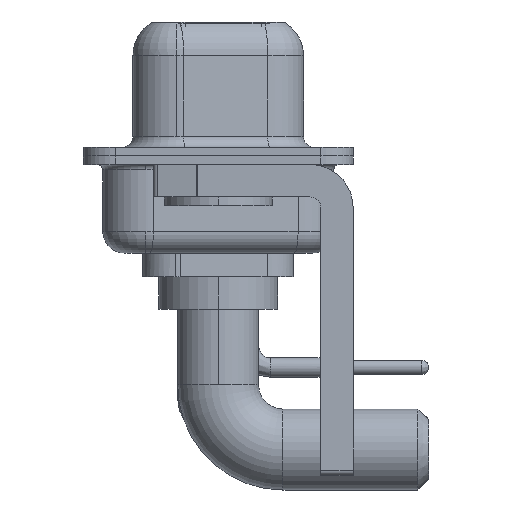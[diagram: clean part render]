
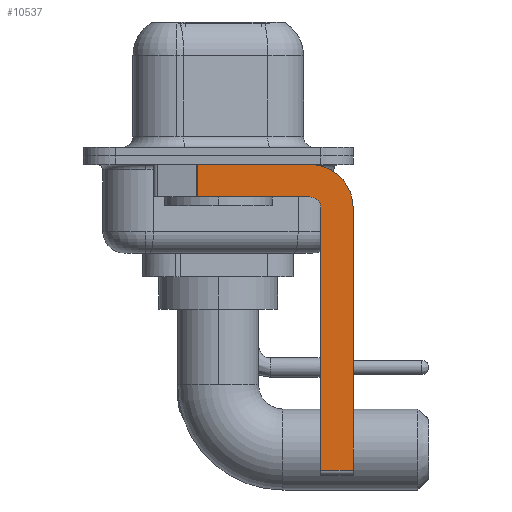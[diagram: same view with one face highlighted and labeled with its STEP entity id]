
A CAD part, left-side view. The second image highlights one B-rep face of the part: STEP entity #10537.
In plain terms, the highlighted planar face has unit normal (-1, 0, 0).
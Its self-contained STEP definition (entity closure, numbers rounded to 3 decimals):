
#95 = DIRECTION ( 'NONE',  ( 0., 0., -1. ) ) ;
#140 = VERTEX_POINT ( 'NONE', #16661 ) ;
#276 = CARTESIAN_POINT ( 'NONE',  ( -2.9, -4.25, -2.4 ) ) ;
#674 = CARTESIAN_POINT ( 'NONE',  ( -2.9, -6.25, -14.55 ) ) ;
#1597 = DIRECTION ( 'NONE',  ( 1., 0., 0. ) ) ;
#1929 = ORIENTED_EDGE ( 'NONE', *, *, #3151, .T. ) ;
#2019 = VECTOR ( 'NONE', #18673, 1000. ) ;
#2050 = EDGE_CURVE ( 'NONE', #140, #2763, #14699, .T. ) ;
#2597 = DIRECTION ( 'NONE',  ( 1., 0., 0. ) ) ;
#2763 = VERTEX_POINT ( 'NONE', #7051 ) ;
#2902 = AXIS2_PLACEMENT_3D ( 'NONE', #276, #18429, #15344 ) ;
#3151 = EDGE_CURVE ( 'NONE', #11367, #9484, #11431, .T. ) ;
#3240 = ORIENTED_EDGE ( 'NONE', *, *, #6135, .F. ) ;
#3324 = CARTESIAN_POINT ( 'NONE',  ( -2.9, -4.25, -14.55 ) ) ;
#4047 = VERTEX_POINT ( 'NONE', #17293 ) ;
#4125 = DIRECTION ( 'NONE',  ( 0., -1., 0. ) ) ;
#4129 = DIRECTION ( 'NONE',  ( 0., 1., 0. ) ) ;
#4454 = CARTESIAN_POINT ( 'NONE',  ( -2.9, -6.25, -2.4 ) ) ;
#4576 = VECTOR ( 'NONE', #4129, 1000. ) ;
#5294 = CARTESIAN_POINT ( 'NONE',  ( -2.9, -4.25, -1.9 ) ) ;
#5442 = LINE ( 'NONE', #17672, #14476 ) ;
#5616 = CARTESIAN_POINT ( 'NONE',  ( -2.9, -4.25, -2.4 ) ) ;
#5773 = VERTEX_POINT ( 'NONE', #9544 ) ;
#5846 = LINE ( 'NONE', #14773, #4576 ) ;
#6135 = EDGE_CURVE ( 'NONE', #4047, #9531, #18574, .T. ) ;
#6260 = CARTESIAN_POINT ( 'NONE',  ( -2.9, -4.75, -14.8 ) ) ;
#6534 = FACE_OUTER_BOUND ( 'NONE', #8795, .T. ) ;
#7051 = CARTESIAN_POINT ( 'NONE',  ( -2.9, -6.25, -2.4 ) ) ;
#7273 = EDGE_CURVE ( 'NONE', #5773, #140, #5442, .T. ) ;
#7577 = ORIENTED_EDGE ( 'NONE', *, *, #19561, .T. ) ;
#8176 = VERTEX_POINT ( 'NONE', #13097 ) ;
#8284 = VECTOR ( 'NONE', #15480, 1000. ) ;
#8582 = EDGE_CURVE ( 'NONE', #9531, #8176, #5846, .T. ) ;
#8728 = DIRECTION ( 'NONE',  ( 0., 0., -1. ) ) ;
#8783 = ORIENTED_EDGE ( 'NONE', *, *, #7273, .F. ) ;
#8795 = EDGE_LOOP ( 'NONE', ( #8783, #7577, #11007, #3240, #8877, #1929, #18086, #10152 ) ) ;
#8877 = ORIENTED_EDGE ( 'NONE', *, *, #10077, .F. ) ;
#9484 = VERTEX_POINT ( 'NONE', #674 ) ;
#9531 = VERTEX_POINT ( 'NONE', #5294 ) ;
#9544 = CARTESIAN_POINT ( 'NONE',  ( -2.9, 0.978, -0.4 ) ) ;
#10077 = EDGE_CURVE ( 'NONE', #11367, #4047, #15580, .T. ) ;
#10152 = ORIENTED_EDGE ( 'NONE', *, *, #2050, .F. ) ;
#10466 = VECTOR ( 'NONE', #11986, 1000. ) ;
#10537 = ADVANCED_FACE ( 'NONE', ( #6534 ), #17246, .F. ) ;
#11007 = ORIENTED_EDGE ( 'NONE', *, *, #8582, .F. ) ;
#11367 = VERTEX_POINT ( 'NONE', #18495 ) ;
#11431 = LINE ( 'NONE', #3324, #8284 ) ;
#11713 = DIRECTION ( 'NONE',  ( 0., 0., -1. ) ) ;
#11986 = DIRECTION ( 'NONE',  ( 0., 0., -1. ) ) ;
#12297 = AXIS2_PLACEMENT_3D ( 'NONE', #15361, #1597, #95 ) ;
#12922 = EDGE_CURVE ( 'NONE', #2763, #9484, #13494, .T. ) ;
#13097 = CARTESIAN_POINT ( 'NONE',  ( -2.9, 0.978, -1.9 ) ) ;
#13494 = LINE ( 'NONE', #4454, #10466 ) ;
#14476 = VECTOR ( 'NONE', #4125, 1000. ) ;
#14699 = CIRCLE ( 'NONE', #16326, 2. ) ;
#14773 = CARTESIAN_POINT ( 'NONE',  ( -2.9, -4.25, -1.9 ) ) ;
#15344 = DIRECTION ( 'NONE',  ( 0., 0., 1. ) ) ;
#15361 = CARTESIAN_POINT ( 'NONE',  ( -2.9, -4.25, -2.4 ) ) ;
#15480 = DIRECTION ( 'NONE',  ( 0., -1., 0. ) ) ;
#15580 = LINE ( 'NONE', #6260, #2019 ) ;
#16326 = AXIS2_PLACEMENT_3D ( 'NONE', #5616, #2597, #8728 ) ;
#16661 = CARTESIAN_POINT ( 'NONE',  ( -2.9, -4.25, -0.4 ) ) ;
#17246 = PLANE ( 'NONE',  #12297 ) ;
#17293 = CARTESIAN_POINT ( 'NONE',  ( -2.9, -4.75, -2.4 ) ) ;
#17672 = CARTESIAN_POINT ( 'NONE',  ( -2.9, 3., -0.4 ) ) ;
#17711 = LINE ( 'NONE', #19305, #19544 ) ;
#18086 = ORIENTED_EDGE ( 'NONE', *, *, #12922, .F. ) ;
#18429 = DIRECTION ( 'NONE',  ( -1., 0., 0. ) ) ;
#18495 = CARTESIAN_POINT ( 'NONE',  ( -2.9, -4.75, -14.55 ) ) ;
#18574 = CIRCLE ( 'NONE', #2902, 0.5 ) ;
#18673 = DIRECTION ( 'NONE',  ( 0., 0., 1. ) ) ;
#19305 = CARTESIAN_POINT ( 'NONE',  ( -2.9, 0.978, -1.9 ) ) ;
#19544 = VECTOR ( 'NONE', #11713, 1000. ) ;
#19561 = EDGE_CURVE ( 'NONE', #5773, #8176, #17711, .T. ) ;
